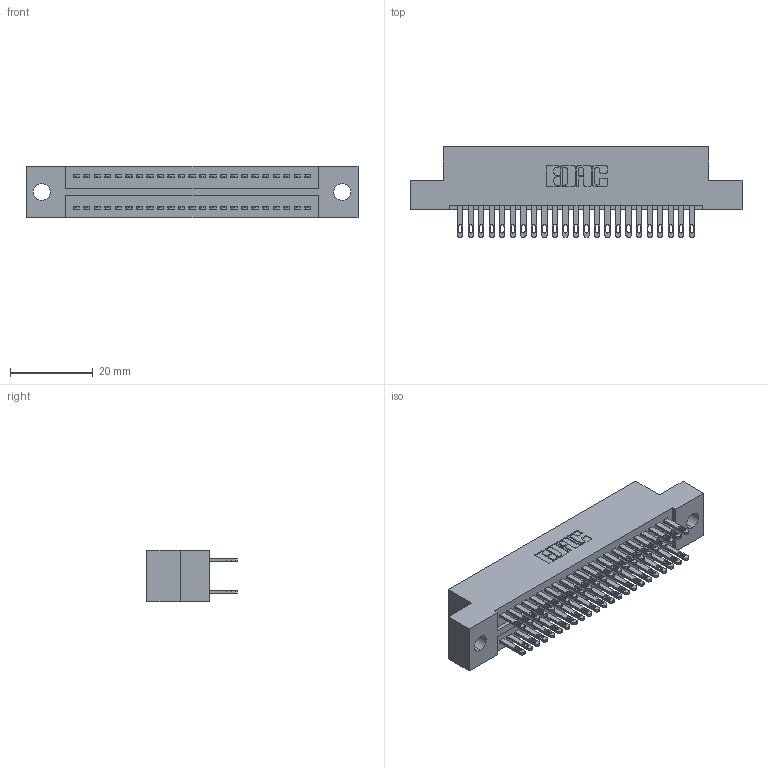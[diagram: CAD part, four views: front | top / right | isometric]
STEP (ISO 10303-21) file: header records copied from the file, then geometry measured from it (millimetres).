
FILE_DESCRIPTION (( 'STEP AP203' ), '1' );
FILE_NAME ('325-046-500-209.STEP', '2020-02-24T22:50:09', ( '' ), ( '' ), 'SwSTEP 2.0', 'SolidWorks 2016', '' );
FILE_SCHEMA (( 'CONFIG_CONTROL_DESIGN' ));
Length unit declared in the file: inch
Products named in the file (3): 325 Part_.160 TH; 325-046-500-209; 325-292-001_325-293-100
Assembly tree (47 placements, depth 2):
  325-046-500-209
    325 Part_.160 TH
    325-292-001_325-293-100  x46
Bounding box: 80.14 x 21.84 x 12.45 mm (x, y, z)
Volume: 10084.6 mm3; surface area: 12156.9 mm2
Topology: 47 solids, 47 shells, 2322 faces, 7073 edges, 4714 vertices
Faces by surface type: plane 1450, cylinder 872
Entity records: 17187 total; most frequent: CARTESIAN_POINT 2870, ORIENTED_EDGE 2806, DIRECTION 2487, EDGE_CURVE 1403, VECTOR 1271, LINE 1271, VERTEX_POINT 934, AXIS2_PLACEMENT_3D 608
